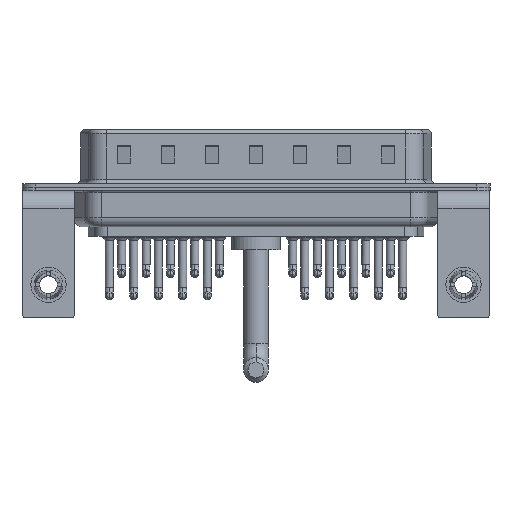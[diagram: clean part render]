
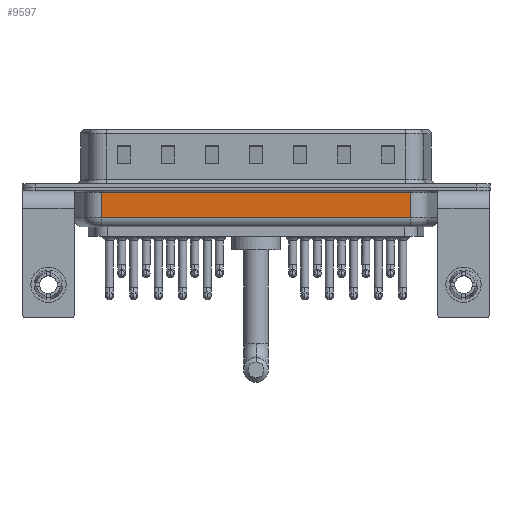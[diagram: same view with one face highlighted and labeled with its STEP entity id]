
A CAD part, front view. The second image highlights one B-rep face of the part: STEP entity #9597.
In plain terms, the highlighted planar face has unit normal (0, -1, 0).
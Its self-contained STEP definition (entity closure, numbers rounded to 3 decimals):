
#292 = EDGE_LOOP ( 'NONE', ( #16092, #14061, #27993, #23984 ) ) ;
#1369 = VERTEX_POINT ( 'NONE', #6573 ) ;
#1615 = FACE_OUTER_BOUND ( 'NONE', #292, .T. ) ;
#1904 = LINE ( 'NONE', #26077, #24934 ) ;
#2009 = CARTESIAN_POINT ( 'NONE',  ( 6.006, -5.35, -3.5 ) ) ;
#3824 = CARTESIAN_POINT ( 'NONE',  ( 6.006, -5.35, -3.5 ) ) ;
#4032 = EDGE_CURVE ( 'NONE', #16115, #1369, #17057, .T. ) ;
#4923 = DIRECTION ( 'NONE',  ( 0., 0., 1. ) ) ;
#6573 = CARTESIAN_POINT ( 'NONE',  ( 41.044, -5.35, -3.5 ) ) ;
#9532 = CARTESIAN_POINT ( 'NONE',  ( 41.044, -5.35, -4.5 ) ) ;
#9597 = ADVANCED_FACE ( 'NONE', ( #1615 ), #10402, .F. ) ;
#10402 = PLANE ( 'NONE',  #15087 ) ;
#11558 = EDGE_CURVE ( 'NONE', #26749, #13947, #20449, .T. ) ;
#12438 = VECTOR ( 'NONE', #21381, 1000. ) ;
#12881 = CARTESIAN_POINT ( 'NONE',  ( 6.006, -5.35, -0.65 ) ) ;
#13695 = CARTESIAN_POINT ( 'NONE',  ( 6.006, -5.35, -0.65 ) ) ;
#13846 = DIRECTION ( 'NONE',  ( -1., 0., 0. ) ) ;
#13947 = VERTEX_POINT ( 'NONE', #12881 ) ;
#14061 = ORIENTED_EDGE ( 'NONE', *, *, #4032, .T. ) ;
#14131 = LINE ( 'NONE', #9532, #22410 ) ;
#15087 = AXIS2_PLACEMENT_3D ( 'NONE', #25939, #21339, #27954 ) ;
#16092 = ORIENTED_EDGE ( 'NONE', *, *, #21507, .F. ) ;
#16115 = VERTEX_POINT ( 'NONE', #2009 ) ;
#17057 = LINE ( 'NONE', #3824, #12438 ) ;
#19158 = CARTESIAN_POINT ( 'NONE',  ( 41.044, -5.35, -0.65 ) ) ;
#20449 = LINE ( 'NONE', #13695, #20951 ) ;
#20951 = VECTOR ( 'NONE', #13846, 1000. ) ;
#21339 = DIRECTION ( 'NONE',  ( 0., 1., 0. ) ) ;
#21381 = DIRECTION ( 'NONE',  ( 1., 0., 0. ) ) ;
#21507 = EDGE_CURVE ( 'NONE', #16115, #13947, #1904, .T. ) ;
#22410 = VECTOR ( 'NONE', #4923, 1000. ) ;
#23930 = DIRECTION ( 'NONE',  ( 0., 0., 1. ) ) ;
#23984 = ORIENTED_EDGE ( 'NONE', *, *, #11558, .T. ) ;
#24335 = EDGE_CURVE ( 'NONE', #1369, #26749, #14131, .T. ) ;
#24934 = VECTOR ( 'NONE', #23930, 1000. ) ;
#25939 = CARTESIAN_POINT ( 'NONE',  ( 6.006, -5.35, -4.5 ) ) ;
#26077 = CARTESIAN_POINT ( 'NONE',  ( 6.006, -5.35, -4.5 ) ) ;
#26749 = VERTEX_POINT ( 'NONE', #19158 ) ;
#27954 = DIRECTION ( 'NONE',  ( 0., 0., 1. ) ) ;
#27993 = ORIENTED_EDGE ( 'NONE', *, *, #24335, .T. ) ;
